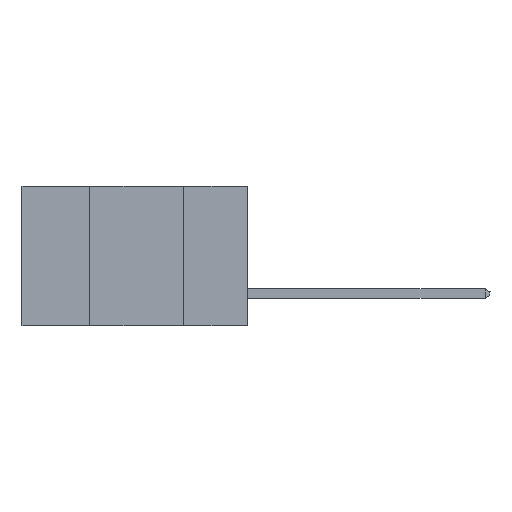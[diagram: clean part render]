
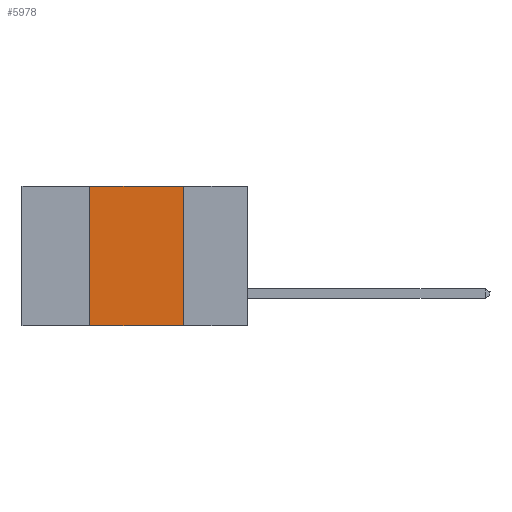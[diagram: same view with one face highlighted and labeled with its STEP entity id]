
A CAD part, left-side view. The second image highlights one B-rep face of the part: STEP entity #5978.
In plain terms, the highlighted planar face has unit normal (-1, 0, 0).
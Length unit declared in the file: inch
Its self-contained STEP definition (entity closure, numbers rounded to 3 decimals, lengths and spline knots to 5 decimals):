
#55 = LINE ( 'NONE', #5615, #210 ) ;
#210 = VECTOR ( 'NONE', #22199, 39.37008 ) ;
#2728 = EDGE_CURVE ( 'NONE', #19110, #11187, #21124, .T. ) ;
#3474 = VECTOR ( 'NONE', #3964, 39.37008 ) ;
#3964 = DIRECTION ( 'NONE',  ( 0., -1., 0. ) ) ;
#4471 = VECTOR ( 'NONE', #13480, 39.37008 ) ;
#4562 = EDGE_CURVE ( 'NONE', #11556, #11187, #9612, .T. ) ;
#4623 = ORIENTED_EDGE ( 'NONE', *, *, #15972, .F. ) ;
#5615 = CARTESIAN_POINT ( 'NONE',  ( 0., 0.42, -0.37 ) ) ;
#5978 = ADVANCED_FACE ( 'NONE', ( #8775 ), #16158, .F. ) ;
#6104 = CARTESIAN_POINT ( 'NONE',  ( 0., 0.6, -0.37 ) ) ;
#8775 = FACE_OUTER_BOUND ( 'NONE', #17561, .T. ) ;
#8954 = CARTESIAN_POINT ( 'NONE',  ( 0., 0.17, 0. ) ) ;
#9419 = EDGE_CURVE ( 'NONE', #11556, #12805, #55, .T. ) ;
#9612 = LINE ( 'NONE', #6104, #4471 ) ;
#11151 = ORIENTED_EDGE ( 'NONE', *, *, #2728, .F. ) ;
#11187 = VERTEX_POINT ( 'NONE', #18317 ) ;
#11275 = DIRECTION ( 'NONE',  ( 0., 0., -1. ) ) ;
#11556 = VERTEX_POINT ( 'NONE', #16584 ) ;
#12805 = VERTEX_POINT ( 'NONE', #20365 ) ;
#13178 = CARTESIAN_POINT ( 'NONE',  ( 0., 0.6, 0. ) ) ;
#13480 = DIRECTION ( 'NONE',  ( 0., -1., 0. ) ) ;
#14232 = ORIENTED_EDGE ( 'NONE', *, *, #9419, .F. ) ;
#15972 = EDGE_CURVE ( 'NONE', #12805, #19110, #18749, .T. ) ;
#16158 = PLANE ( 'NONE',  #19233 ) ;
#16584 = CARTESIAN_POINT ( 'NONE',  ( 0., 0.42, -0.37 ) ) ;
#17561 = EDGE_LOOP ( 'NONE', ( #11151, #4623, #14232, #20491 ) ) ;
#18317 = CARTESIAN_POINT ( 'NONE',  ( 0., 0.17, -0.37 ) ) ;
#18733 = VECTOR ( 'NONE', #21622, 39.37008 ) ;
#18749 = LINE ( 'NONE', #13178, #3474 ) ;
#19110 = VERTEX_POINT ( 'NONE', #8954 ) ;
#19233 = AXIS2_PLACEMENT_3D ( 'NONE', #23534, #22302, #11275 ) ;
#19320 = CARTESIAN_POINT ( 'NONE',  ( 0., 0.17, -0.37 ) ) ;
#20365 = CARTESIAN_POINT ( 'NONE',  ( 0., 0.42, 0. ) ) ;
#20491 = ORIENTED_EDGE ( 'NONE', *, *, #4562, .T. ) ;
#21124 = LINE ( 'NONE', #19320, #18733 ) ;
#21622 = DIRECTION ( 'NONE',  ( 0., 0., -1. ) ) ;
#22199 = DIRECTION ( 'NONE',  ( 0., 0., 1. ) ) ;
#22302 = DIRECTION ( 'NONE',  ( 1., 0., 0. ) ) ;
#23534 = CARTESIAN_POINT ( 'NONE',  ( 0., 0.6, 0. ) ) ;
